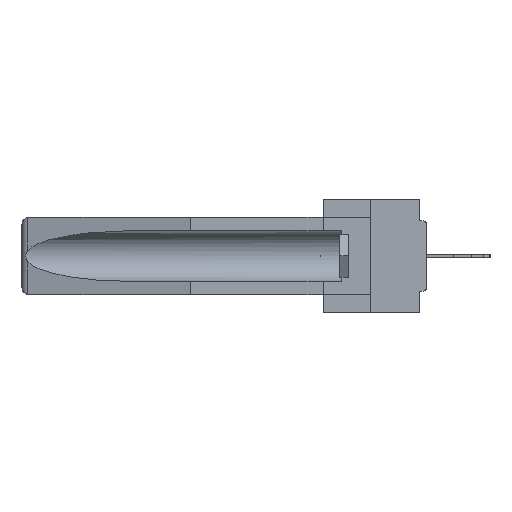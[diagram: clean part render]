
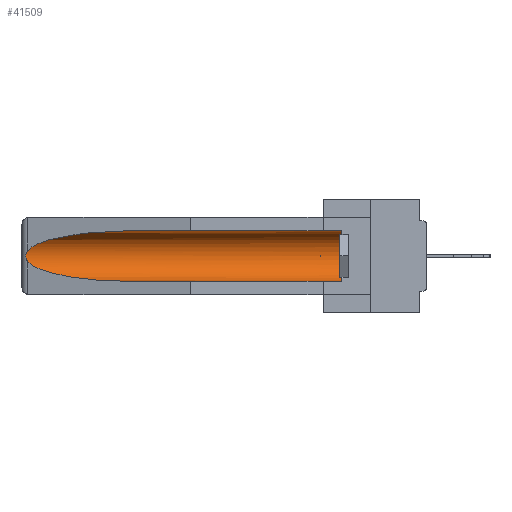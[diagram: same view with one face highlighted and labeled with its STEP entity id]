
A CAD part, left-side view. The second image highlights one B-rep face of the part: STEP entity #41509.
In plain terms, the highlighted cylindrical face has radius 2.857 mm (diameter 5.715 mm), a partial arc.
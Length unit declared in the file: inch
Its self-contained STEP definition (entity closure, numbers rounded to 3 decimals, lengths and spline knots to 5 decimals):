
#10 = ORIENTED_EDGE ( 'NONE', *, *, #6326, .T. ) ;
#731 = EDGE_LOOP ( 'NONE', ( #17016, #12994, #8136, #21339, #26956, #10 ) ) ;
#990 = CARTESIAN_POINT ( 'NONE',  ( 0.155, 1.07973, -0.284 ) ) ;
#1249 = CARTESIAN_POINT ( 'NONE',  ( 0.26654, 1.53092, -0.15636 ) ) ;
#2415 = CARTESIAN_POINT ( 'NONE',  ( 0.26537, 1.52718, -0.19328 ) ) ;
#3177 = CARTESIAN_POINT ( 'NONE',  ( 0.26537, 1.52718, -0.14972 ) ) ;
#3916 = VERTEX_POINT ( 'NONE', #990 ) ;
#4027 = CARTESIAN_POINT ( 'NONE',  ( 0.2673, 1.5327, -0.16383 ) ) ;
#6033 = DIRECTION ( 'NONE',  ( 0., 1., 0. ) ) ;
#6326 = EDGE_CURVE ( 'NONE', #26221, #40408, #31585, .T. ) ;
#6539 = CARTESIAN_POINT ( 'NONE',  ( 0.155, -0.30754, -0.1715 ) ) ;
#6963 = DIRECTION ( 'NONE',  ( 0., 1., 0. ) ) ;
#7210 = CARTESIAN_POINT ( 'NONE',  ( 0.26537, 1.52718, -0.14972 ) ) ;
#7508 = EDGE_CURVE ( 'NONE', #40830, #39257, #31763, .T. ) ;
#7624 = CARTESIAN_POINT ( 'NONE',  ( 0.26655, 1.53094, -0.18657 ) ) ;
#7732 = CARTESIAN_POINT ( 'NONE',  ( 0.26537, 1.52718, -0.14972 ) ) ;
#8136 = ORIENTED_EDGE ( 'NONE', *, *, #15455, .T. ) ;
#8299 = DIRECTION ( 'NONE',  ( 0., 0., 1. ) ) ;
#9721 = CARTESIAN_POINT ( 'NONE',  ( 0.155, 1.07973, -0.059 ) ) ;
#10619 = DIRECTION ( 'NONE',  ( 0., -1., 0. ) ) ;
#10977 = LINE ( 'NONE', #33398, #14219 ) ;
#11229 = CARTESIAN_POINT ( 'NONE',  ( 0.155, 0.126, -0.1715 ) ) ;
#12994 = ORIENTED_EDGE ( 'NONE', *, *, #7508, .T. ) ;
#13714 = CARTESIAN_POINT ( 'NONE',  ( 0.2675, 1.53308, -0.17534 ) ) ;
#14219 = VECTOR ( 'NONE', #17918, 39.37008 ) ;
#15168 = CARTESIAN_POINT ( 'NONE',  ( 0.21114, 1.30732, -0.284 ) ) ;
#15455 = EDGE_CURVE ( 'NONE', #39257, #3916, #38519, .T. ) ;
#16429 = FACE_OUTER_BOUND ( 'NONE', #731, .T. ) ;
#16867 = CARTESIAN_POINT ( 'NONE',  ( 0.2675, 1.53308, -0.16763 ) ) ;
#17016 = ORIENTED_EDGE ( 'NONE', *, *, #17776, .T. ) ;
#17512 = CIRCLE ( 'NONE', #23611, 0.1125 ) ;
#17776 = EDGE_CURVE ( 'NONE', #40408, #40830, #26866, .T. ) ;
#17918 = DIRECTION ( 'NONE',  ( 0., 1., 0. ) ) ;
#17921 = CARTESIAN_POINT ( 'NONE',  ( 0.155, 0.126, -0.059 ) ) ;
#20044 = CARTESIAN_POINT ( 'NONE',  ( 0.26597, 1.52961, -0.15275 ) ) ;
#20474 = CARTESIAN_POINT ( 'NONE',  ( 0.26597, 1.5296, -0.19026 ) ) ;
#20803 = VECTOR ( 'NONE', #6033, 39.37008 ) ;
#21294 = CARTESIAN_POINT ( 'NONE',  ( 0.25451, 1.48313, -0.24835 ) ) ;
#21339 = ORIENTED_EDGE ( 'NONE', *, *, #41106, .F. ) ;
#22118 = CARTESIAN_POINT ( 'NONE',  ( 0.21114, 1.30732, -0.059 ) ) ;
#22778 = CARTESIAN_POINT ( 'NONE',  ( 0.155, 0.126, -0.284 ) ) ;
#23611 = AXIS2_PLACEMENT_3D ( 'NONE', #11229, #10619, #8299 ) ;
#24179 = CARTESIAN_POINT ( 'NONE',  ( 0.155, 1.07973, -0.059 ) ) ;
#25250 = CARTESIAN_POINT ( 'NONE',  ( 0.155, -0.30754, -0.059 ) ) ;
#26221 = VERTEX_POINT ( 'NONE', #17921 ) ;
#26866 =( BOUNDED_CURVE ( )  B_SPLINE_CURVE ( 3, ( #9721, #22118, #31897, #3177 ),
 .UNSPECIFIED., .F., .F. ) 
 B_SPLINE_CURVE_WITH_KNOTS ( ( 4, 4 ),
 ( 4.71239, 6.08839 ),
 .UNSPECIFIED. ) 
 CURVE ( )  GEOMETRIC_REPRESENTATION_ITEM ( )  RATIONAL_B_SPLINE_CURVE ( ( 1., 0.848, 0.848, 1. ) ) 
 REPRESENTATION_ITEM ( '' )  );
#26956 = ORIENTED_EDGE ( 'NONE', *, *, #30220, .T. ) ;
#27734 = AXIS2_PLACEMENT_3D ( 'NONE', #6539, #6963, #29113 ) ;
#29113 = DIRECTION ( 'NONE',  ( 0., 0., 1. ) ) ;
#29337 = CYLINDRICAL_SURFACE ( 'NONE', #27734, 0.1125 ) ;
#30220 = EDGE_CURVE ( 'NONE', #38566, #26221, #17512, .T. ) ;
#31585 = LINE ( 'NONE', #25250, #20803 ) ;
#31763 = B_SPLINE_CURVE_WITH_KNOTS ( 'NONE', 3,
 ( #7210, #20044, #1249, #4027, #16867, #13714, #36559, #7624, #20474, #33395 ),
 .UNSPECIFIED., .F., .F.,
 ( 4, 2, 2, 2, 4 ),
 ( 0., 0.00029, 0.00058, 0.00087, 0.00117 ),
 .UNSPECIFIED. ) ;
#31897 = CARTESIAN_POINT ( 'NONE',  ( 0.25451, 1.48313, -0.09465 ) ) ;
#33395 = CARTESIAN_POINT ( 'NONE',  ( 0.26537, 1.52718, -0.19328 ) ) ;
#33398 = CARTESIAN_POINT ( 'NONE',  ( 0.155, -0.30754, -0.284 ) ) ;
#34225 = CARTESIAN_POINT ( 'NONE',  ( 0.155, 1.07973, -0.284 ) ) ;
#36559 = CARTESIAN_POINT ( 'NONE',  ( 0.2673, 1.53269, -0.17917 ) ) ;
#37402 = CARTESIAN_POINT ( 'NONE',  ( 0.26537, 1.52718, -0.19328 ) ) ;
#38519 =( BOUNDED_CURVE ( )  B_SPLINE_CURVE ( 3, ( #37402, #21294, #15168, #34225 ),
 .UNSPECIFIED., .F., .F. ) 
 B_SPLINE_CURVE_WITH_KNOTS ( ( 4, 4 ),
 ( 0.1948, 1.5708 ),
 .UNSPECIFIED. ) 
 CURVE ( )  GEOMETRIC_REPRESENTATION_ITEM ( )  RATIONAL_B_SPLINE_CURVE ( ( 1., 0.848, 0.848, 1. ) ) 
 REPRESENTATION_ITEM ( '' )  );
#38566 = VERTEX_POINT ( 'NONE', #22778 ) ;
#39257 = VERTEX_POINT ( 'NONE', #2415 ) ;
#40408 = VERTEX_POINT ( 'NONE', #24179 ) ;
#40830 = VERTEX_POINT ( 'NONE', #7732 ) ;
#41106 = EDGE_CURVE ( 'NONE', #38566, #3916, #10977, .T. ) ;
#41509 = ADVANCED_FACE ( 'NONE', ( #16429 ), #29337, .F. ) ;
